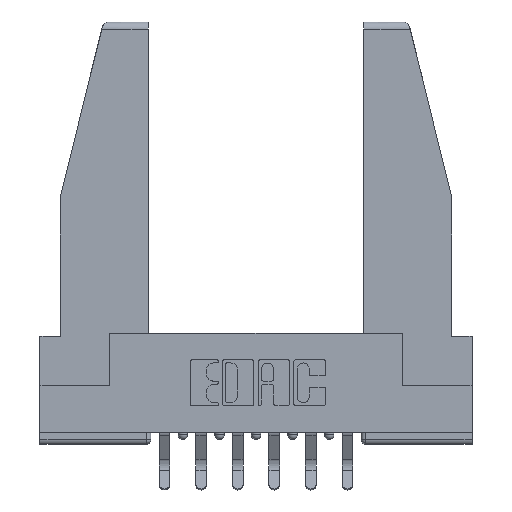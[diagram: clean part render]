
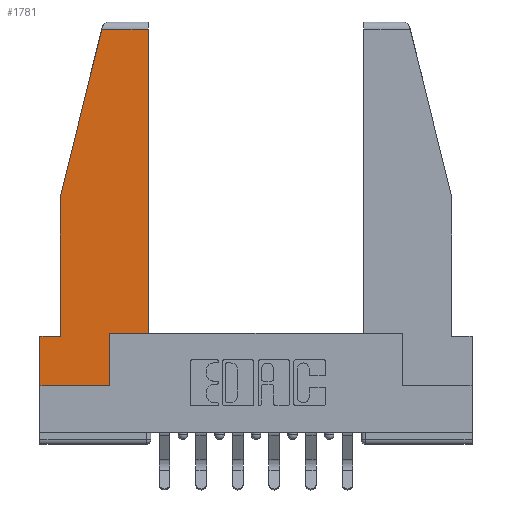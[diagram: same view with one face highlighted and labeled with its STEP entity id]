
A CAD part, top view. The second image highlights one B-rep face of the part: STEP entity #1781.
In plain terms, the highlighted planar face has unit normal (0, 0, 1).
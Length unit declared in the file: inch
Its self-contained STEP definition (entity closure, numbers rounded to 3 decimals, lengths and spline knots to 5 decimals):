
#60 = VERTEX_POINT ( 'NONE', #9593 ) ;
#105 = CARTESIAN_POINT ( 'NONE',  ( 0.271, 1.55, 0. ) ) ;
#112 = CARTESIAN_POINT ( 'NONE',  ( 0., 0., 0. ) ) ;
#162 = CARTESIAN_POINT ( 'NONE',  ( 0., 0., 0. ) ) ;
#199 = ORIENTED_EDGE ( 'NONE', *, *, #1931, .T. ) ;
#307 = CARTESIAN_POINT ( 'NONE',  ( 0., 0., 0. ) ) ;
#404 = VECTOR ( 'NONE', #10697, 39.37008 ) ;
#605 = DIRECTION ( 'NONE',  ( 0., 1., 0. ) ) ;
#841 = EDGE_CURVE ( 'NONE', #9501, #9208, #11579, .T. ) ;
#866 = CARTESIAN_POINT ( 'NONE',  ( 0.297, 0., 0. ) ) ;
#952 = CARTESIAN_POINT ( 'NONE',  ( 0.086, 0.21, 0. ) ) ;
#1014 = EDGE_CURVE ( 'NONE', #5022, #5221, #4208, .T. ) ;
#1023 = CARTESIAN_POINT ( 'NONE',  ( 0., 0.21, 0. ) ) ;
#1077 = ORIENTED_EDGE ( 'NONE', *, *, #11321, .T. ) ;
#1191 = CARTESIAN_POINT ( 'NONE',  ( 0.297, 0., 0. ) ) ;
#1276 = EDGE_CURVE ( 'NONE', #9331, #1639, #9408, .T. ) ;
#1602 = EDGE_CURVE ( 'NONE', #60, #5022, #7261, .T. ) ;
#1639 = VERTEX_POINT ( 'NONE', #8255 ) ;
#1781 = ADVANCED_FACE ( 'NONE', ( #4042 ), #11471, .T. ) ;
#1931 = EDGE_CURVE ( 'NONE', #1639, #60, #7132, .T. ) ;
#1996 = DIRECTION ( 'NONE',  ( 1., 0., 0. ) ) ;
#2036 = EDGE_CURVE ( 'NONE', #11683, #2670, #10085, .T. ) ;
#2116 = VECTOR ( 'NONE', #12190, 39.37008 ) ;
#2234 = CARTESIAN_POINT ( 'NONE',  ( 0.2636, 1.52, 0. ) ) ;
#2298 = DIRECTION ( 'NONE',  ( 1., 0., 0. ) ) ;
#2314 = ORIENTED_EDGE ( 'NONE', *, *, #1014, .T. ) ;
#2670 = VERTEX_POINT ( 'NONE', #952 ) ;
#2856 = DIRECTION ( 'NONE',  ( 0., 0., 1. ) ) ;
#3004 = LINE ( 'NONE', #307, #7626 ) ;
#3118 = ORIENTED_EDGE ( 'NONE', *, *, #2036, .T. ) ;
#3171 = DIRECTION ( 'NONE',  ( -0.239, -0.971, 0. ) ) ;
#3531 = EDGE_LOOP ( 'NONE', ( #5145, #2314, #5935, #3118, #1077, #7485, #5298, #9884, #199 ) ) ;
#3715 = CARTESIAN_POINT ( 'NONE',  ( 0.086, 0.8, 0. ) ) ;
#4024 = CARTESIAN_POINT ( 'NONE',  ( 0., 1.52, 0. ) ) ;
#4042 = FACE_OUTER_BOUND ( 'NONE', #3531, .T. ) ;
#4067 = DIRECTION ( 'NONE',  ( 1., 0., 0. ) ) ;
#4208 = LINE ( 'NONE', #4024, #404 ) ;
#4642 = CARTESIAN_POINT ( 'NONE',  ( 0.086, 0.8, 0. ) ) ;
#4715 = LINE ( 'NONE', #4781, #12091 ) ;
#4781 = CARTESIAN_POINT ( 'NONE',  ( 0., 0.21, 0. ) ) ;
#5022 = VERTEX_POINT ( 'NONE', #10402 ) ;
#5145 = ORIENTED_EDGE ( 'NONE', *, *, #1602, .T. ) ;
#5221 = VERTEX_POINT ( 'NONE', #2234 ) ;
#5298 = ORIENTED_EDGE ( 'NONE', *, *, #6033, .T. ) ;
#5935 = ORIENTED_EDGE ( 'NONE', *, *, #9754, .T. ) ;
#6033 = EDGE_CURVE ( 'NONE', #9208, #9331, #3004, .T. ) ;
#7132 = LINE ( 'NONE', #10782, #10287 ) ;
#7261 = LINE ( 'NONE', #7320, #10143 ) ;
#7320 = CARTESIAN_POINT ( 'NONE',  ( 0.461, 0.223, 0. ) ) ;
#7485 = ORIENTED_EDGE ( 'NONE', *, *, #841, .T. ) ;
#7495 = DIRECTION ( 'NONE',  ( 0., -1., 0. ) ) ;
#7626 = VECTOR ( 'NONE', #4067, 39.37008 ) ;
#8255 = CARTESIAN_POINT ( 'NONE',  ( 0.297, 0.223, 0. ) ) ;
#8562 = VECTOR ( 'NONE', #7495, 39.37008 ) ;
#8651 = LINE ( 'NONE', #105, #8713 ) ;
#8713 = VECTOR ( 'NONE', #3171, 39.37008 ) ;
#9208 = VERTEX_POINT ( 'NONE', #112 ) ;
#9331 = VERTEX_POINT ( 'NONE', #1191 ) ;
#9408 = LINE ( 'NONE', #866, #11590 ) ;
#9501 = VERTEX_POINT ( 'NONE', #10981 ) ;
#9593 = CARTESIAN_POINT ( 'NONE',  ( 0.461, 0.223, 0. ) ) ;
#9754 = EDGE_CURVE ( 'NONE', #5221, #11683, #8651, .T. ) ;
#9884 = ORIENTED_EDGE ( 'NONE', *, *, #1276, .T. ) ;
#10085 = LINE ( 'NONE', #3715, #2116 ) ;
#10143 = VECTOR ( 'NONE', #605, 39.37008 ) ;
#10287 = VECTOR ( 'NONE', #2298, 39.37008 ) ;
#10402 = CARTESIAN_POINT ( 'NONE',  ( 0.461, 1.52, 0. ) ) ;
#10697 = DIRECTION ( 'NONE',  ( -1., 0., 0. ) ) ;
#10731 = DIRECTION ( 'NONE',  ( 0., 1., 0. ) ) ;
#10782 = CARTESIAN_POINT ( 'NONE',  ( 0.297, 0.223, 0. ) ) ;
#10981 = CARTESIAN_POINT ( 'NONE',  ( 0., 0.21, 0. ) ) ;
#11321 = EDGE_CURVE ( 'NONE', #2670, #9501, #4715, .T. ) ;
#11471 = PLANE ( 'NONE',  #11782 ) ;
#11579 = LINE ( 'NONE', #1023, #8562 ) ;
#11590 = VECTOR ( 'NONE', #10731, 39.37008 ) ;
#11683 = VERTEX_POINT ( 'NONE', #4642 ) ;
#11782 = AXIS2_PLACEMENT_3D ( 'NONE', #162, #2856, #1996 ) ;
#12091 = VECTOR ( 'NONE', #12327, 39.37008 ) ;
#12190 = DIRECTION ( 'NONE',  ( 0., -1., 0. ) ) ;
#12327 = DIRECTION ( 'NONE',  ( -1., 0., 0. ) ) ;
